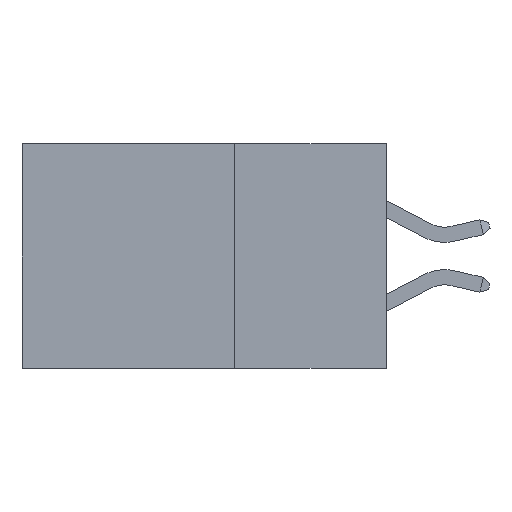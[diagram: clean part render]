
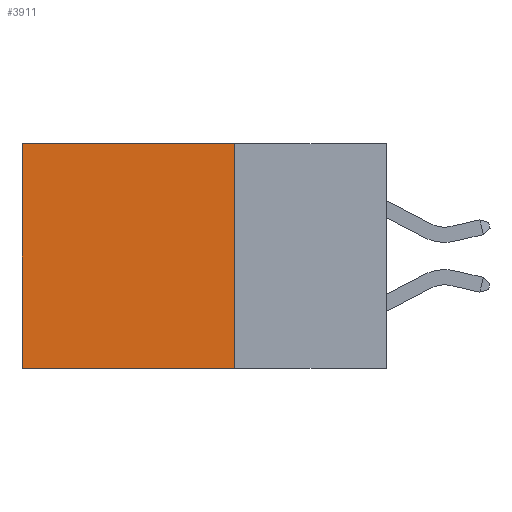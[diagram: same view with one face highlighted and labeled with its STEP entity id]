
A CAD part, left-side view. The second image highlights one B-rep face of the part: STEP entity #3911.
In plain terms, the highlighted planar face has unit normal (-1, 0, 0).
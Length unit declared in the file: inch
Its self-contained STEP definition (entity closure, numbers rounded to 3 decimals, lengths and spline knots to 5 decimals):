
#355 = CARTESIAN_POINT ( 'NONE',  ( 0.2615, 0.25, 0. ) ) ;
#714 = VECTOR ( 'NONE', #16109, 39.37008 ) ;
#1733 = VERTEX_POINT ( 'NONE', #23785 ) ;
#2281 = VECTOR ( 'NONE', #23386, 39.37008 ) ;
#2693 = FACE_OUTER_BOUND ( 'NONE', #7346, .T. ) ;
#3911 = ADVANCED_FACE ( 'NONE', ( #2693 ), #21379, .F. ) ;
#5557 = VECTOR ( 'NONE', #23825, 39.37008 ) ;
#6956 = ORIENTED_EDGE ( 'NONE', *, *, #7896, .T. ) ;
#7346 = EDGE_LOOP ( 'NONE', ( #6956, #18039, #10313, #17325 ) ) ;
#7896 = EDGE_CURVE ( 'NONE', #1733, #19243, #23732, .T. ) ;
#8674 = CARTESIAN_POINT ( 'NONE',  ( 0.2615, 0.25, -0.37 ) ) ;
#9056 = EDGE_CURVE ( 'NONE', #21247, #1733, #10621, .T. ) ;
#9159 = CARTESIAN_POINT ( 'NONE',  ( 0.2615, 0.25, -0.37 ) ) ;
#10313 = ORIENTED_EDGE ( 'NONE', *, *, #21774, .F. ) ;
#10509 = DIRECTION ( 'NONE',  ( 1., 0., 0. ) ) ;
#10621 = LINE ( 'NONE', #23287, #714 ) ;
#11127 = CARTESIAN_POINT ( 'NONE',  ( 0.2615, 0.6, -0.37 ) ) ;
#12028 = LINE ( 'NONE', #21569, #2281 ) ;
#12828 = DIRECTION ( 'NONE',  ( 0., 1., 0. ) ) ;
#13691 = LINE ( 'NONE', #9159, #17970 ) ;
#16109 = DIRECTION ( 'NONE',  ( 0., 1., 0. ) ) ;
#17325 = ORIENTED_EDGE ( 'NONE', *, *, #9056, .T. ) ;
#17457 = AXIS2_PLACEMENT_3D ( 'NONE', #8674, #10509, #23187 ) ;
#17643 = CARTESIAN_POINT ( 'NONE',  ( 0.2615, 0.6, -0.37 ) ) ;
#17970 = VECTOR ( 'NONE', #12828, 39.37008 ) ;
#18039 = ORIENTED_EDGE ( 'NONE', *, *, #22697, .F. ) ;
#19192 = CARTESIAN_POINT ( 'NONE',  ( 0.2615, 0.25, -0.37 ) ) ;
#19243 = VERTEX_POINT ( 'NONE', #17643 ) ;
#21247 = VERTEX_POINT ( 'NONE', #355 ) ;
#21379 = PLANE ( 'NONE',  #17457 ) ;
#21569 = CARTESIAN_POINT ( 'NONE',  ( 0.2615, 0.25, -0.37 ) ) ;
#21774 = EDGE_CURVE ( 'NONE', #21247, #22335, #12028, .T. ) ;
#22335 = VERTEX_POINT ( 'NONE', #19192 ) ;
#22697 = EDGE_CURVE ( 'NONE', #22335, #19243, #13691, .T. ) ;
#23187 = DIRECTION ( 'NONE',  ( 0., 0., -1. ) ) ;
#23287 = CARTESIAN_POINT ( 'NONE',  ( 0.2615, 0.25, 0. ) ) ;
#23386 = DIRECTION ( 'NONE',  ( 0., 0., -1. ) ) ;
#23732 = LINE ( 'NONE', #11127, #5557 ) ;
#23785 = CARTESIAN_POINT ( 'NONE',  ( 0.2615, 0.6, 0. ) ) ;
#23825 = DIRECTION ( 'NONE',  ( 0., 0., -1. ) ) ;
